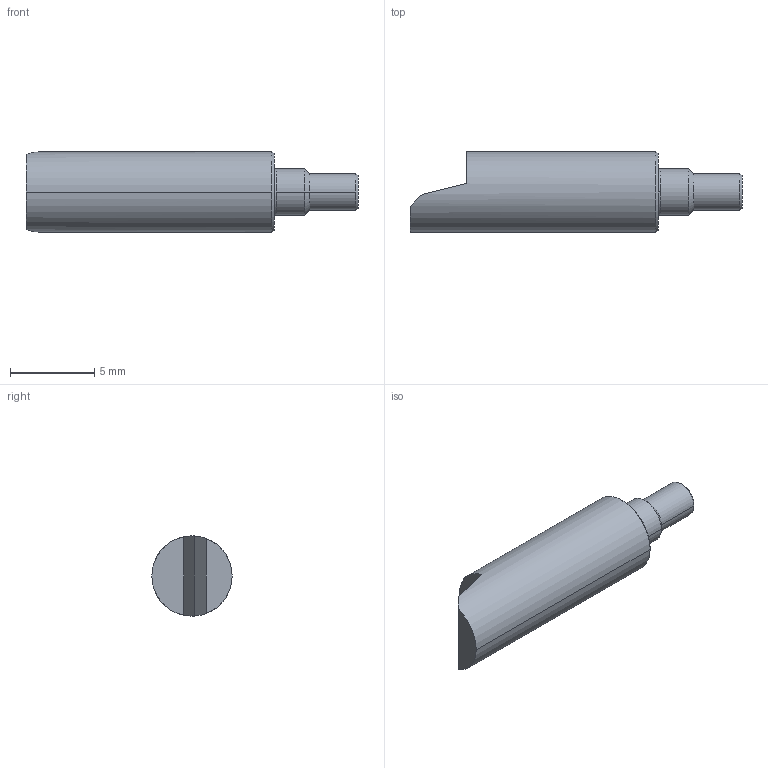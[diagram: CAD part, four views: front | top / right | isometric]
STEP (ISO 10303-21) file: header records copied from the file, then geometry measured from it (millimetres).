
FILE_DESCRIPTION (( 'STEP AP214' ), '1' );
FILE_NAME ('Front Extractor Spring Guide.step', '2014-07-30T19:45:52', ( 'WarFairy' ), ( '' ), 'SwSTEP 2.0', 'SolidWorks 2013', '' );
FILE_SCHEMA (( 'AUTOMOTIVE_DESIGN' ));
Length unit declared in the file: millimetre
Products named in the file (1): Front Extractor Spring Guide
Bounding box: 19.68 x 4.76 x 4.76 mm (x, y, z)
Volume: 255.3 mm3; surface area: 276 mm2
Topology: 1 solids, 1 shells, 20 faces, 43 edges, 26 vertices
Faces by surface type: cone 6, cylinder 6, plane 6, torus 2
Entity records: 581 total; most frequent: DIRECTION 105, CARTESIAN_POINT 102, ORIENTED_EDGE 86, AXIS2_PLACEMENT_3D 45, EDGE_CURVE 43, VERTEX_POINT 26, CIRCLE 24, EDGE_LOOP 21
